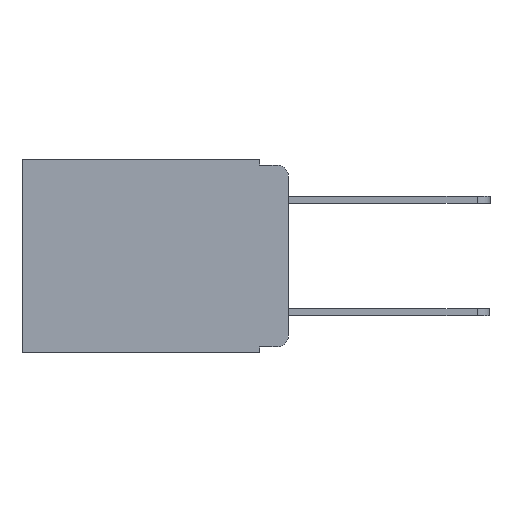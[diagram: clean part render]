
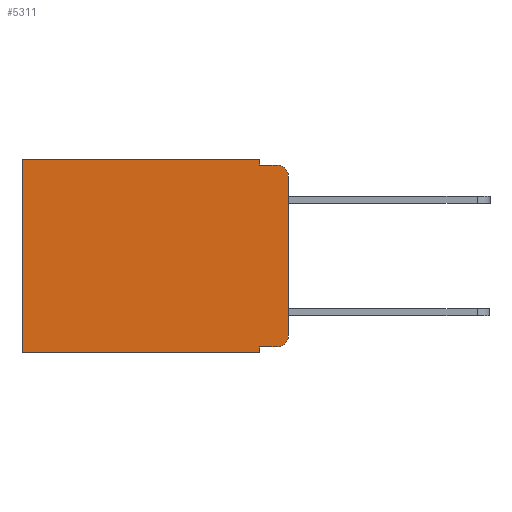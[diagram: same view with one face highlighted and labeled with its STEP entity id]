
A CAD part, left-side view. The second image highlights one B-rep face of the part: STEP entity #5311.
In plain terms, the highlighted planar face has unit normal (-1, 0, 0).
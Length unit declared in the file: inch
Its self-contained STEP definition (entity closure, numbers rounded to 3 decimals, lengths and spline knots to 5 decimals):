
#105 = ORIENTED_EDGE ( 'NONE', *, *, #3213, .T. ) ;
#122 = CARTESIAN_POINT ( 'NONE',  ( 0.298, 0.02, -0.333 ) ) ;
#184 = ORIENTED_EDGE ( 'NONE', *, *, #7238, .F. ) ;
#425 = ORIENTED_EDGE ( 'NONE', *, *, #9780, .T. ) ;
#528 = CARTESIAN_POINT ( 'NONE',  ( 0.298, 0.051, 0. ) ) ;
#529 = DIRECTION ( 'NONE',  ( 0., 0., -1. ) ) ;
#552 = ORIENTED_EDGE ( 'NONE', *, *, #8776, .F. ) ;
#655 = DIRECTION ( 'NONE',  ( 0., 0., -1. ) ) ;
#945 = ORIENTED_EDGE ( 'NONE', *, *, #9925, .T. ) ;
#1077 = ORIENTED_EDGE ( 'NONE', *, *, #9203, .F. ) ;
#1279 = VECTOR ( 'NONE', #6549, 39.37008 ) ;
#1301 = VECTOR ( 'NONE', #7329, 39.37008 ) ;
#1614 = EDGE_CURVE ( 'NONE', #9041, #2381, #5619, .T. ) ;
#1632 = LINE ( 'NONE', #2335, #6495 ) ;
#1778 = VERTEX_POINT ( 'NONE', #10409 ) ;
#2032 = LINE ( 'NONE', #11807, #4285 ) ;
#2217 = VERTEX_POINT ( 'NONE', #7768 ) ;
#2334 = ORIENTED_EDGE ( 'NONE', *, *, #5636, .T. ) ;
#2335 = CARTESIAN_POINT ( 'NONE',  ( 0.298, 0.051, 0. ) ) ;
#2381 = VERTEX_POINT ( 'NONE', #10633 ) ;
#2406 = AXIS2_PLACEMENT_3D ( 'NONE', #9473, #9504, #4091 ) ;
#2476 = VECTOR ( 'NONE', #6270, 39.37008 ) ;
#2969 = ORIENTED_EDGE ( 'NONE', *, *, #1614, .F. ) ;
#2972 = ORIENTED_EDGE ( 'NONE', *, *, #9339, .F. ) ;
#3111 = LINE ( 'NONE', #8207, #10312 ) ;
#3213 = EDGE_CURVE ( 'NONE', #12043, #4428, #3964, .T. ) ;
#3323 = DIRECTION ( 'NONE',  ( 0., 0., -1. ) ) ;
#3486 = CARTESIAN_POINT ( 'NONE',  ( 0.298, 0., 0. ) ) ;
#3513 = CIRCLE ( 'NONE', #10427, 0.02 ) ;
#3964 = LINE ( 'NONE', #3486, #1279 ) ;
#3982 = LINE ( 'NONE', #528, #1301 ) ;
#4091 = DIRECTION ( 'NONE',  ( 0., 0., -1. ) ) ;
#4285 = VECTOR ( 'NONE', #4687, 39.37008 ) ;
#4428 = VERTEX_POINT ( 'NONE', #7315 ) ;
#4435 = DIRECTION ( 'NONE',  ( 0., 1., 0. ) ) ;
#4531 = CARTESIAN_POINT ( 'NONE',  ( 0.298, 0.02, -0.03 ) ) ;
#4687 = DIRECTION ( 'NONE',  ( 0., -1., 0. ) ) ;
#5068 = CARTESIAN_POINT ( 'NONE',  ( 0.298, 0.051, -0.343 ) ) ;
#5310 = LINE ( 'NONE', #9744, #2476 ) ;
#5311 = ADVANCED_FACE ( 'NONE', ( #10951 ), #12104, .F. ) ;
#5364 = AXIS2_PLACEMENT_3D ( 'NONE', #11672, #6459, #529 ) ;
#5519 = DIRECTION ( 'NONE',  ( 0., 0., -1. ) ) ;
#5619 = LINE ( 'NONE', #6500, #10027 ) ;
#5636 = EDGE_CURVE ( 'NONE', #11050, #2381, #10247, .T. ) ;
#6270 = DIRECTION ( 'NONE',  ( 0., 0., -1. ) ) ;
#6459 = DIRECTION ( 'NONE',  ( -1., 0., 0. ) ) ;
#6495 = VECTOR ( 'NONE', #3323, 39.37008 ) ;
#6500 = CARTESIAN_POINT ( 'NONE',  ( 0.298, 0., 0. ) ) ;
#6549 = DIRECTION ( 'NONE',  ( 0., 1., 0. ) ) ;
#7211 = CARTESIAN_POINT ( 'NONE',  ( 0.298, 0., -0.343 ) ) ;
#7238 = EDGE_CURVE ( 'NONE', #9681, #12063, #8993, .T. ) ;
#7286 = CARTESIAN_POINT ( 'NONE',  ( 0.298, 0.051, 0. ) ) ;
#7315 = CARTESIAN_POINT ( 'NONE',  ( 0.298, 0.473, 0. ) ) ;
#7329 = DIRECTION ( 'NONE',  ( 0., 0., -1. ) ) ;
#7437 = EDGE_CURVE ( 'NONE', #2217, #11050, #2032, .T. ) ;
#7768 = CARTESIAN_POINT ( 'NONE',  ( 0.298, 0.051, -0.333 ) ) ;
#8171 = CARTESIAN_POINT ( 'NONE',  ( 0.298, 0.473, -0.343 ) ) ;
#8207 = CARTESIAN_POINT ( 'NONE',  ( 0.298, 0.051, -0.01 ) ) ;
#8595 = ORIENTED_EDGE ( 'NONE', *, *, #7437, .T. ) ;
#8776 = EDGE_CURVE ( 'NONE', #12043, #9581, #3982, .T. ) ;
#8993 = LINE ( 'NONE', #7211, #11037 ) ;
#9041 = VERTEX_POINT ( 'NONE', #9429 ) ;
#9203 = EDGE_CURVE ( 'NONE', #2217, #9681, #1632, .T. ) ;
#9339 = EDGE_CURVE ( 'NONE', #9581, #1778, #3111, .T. ) ;
#9429 = CARTESIAN_POINT ( 'NONE',  ( 0.298, 0., -0.03 ) ) ;
#9473 = CARTESIAN_POINT ( 'NONE',  ( 0.298, 0., 0. ) ) ;
#9504 = DIRECTION ( 'NONE',  ( 1., 0., 0. ) ) ;
#9581 = VERTEX_POINT ( 'NONE', #11181 ) ;
#9681 = VERTEX_POINT ( 'NONE', #5068 ) ;
#9744 = CARTESIAN_POINT ( 'NONE',  ( 0.298, 0.473, 0. ) ) ;
#9780 = EDGE_CURVE ( 'NONE', #4428, #12063, #5310, .T. ) ;
#9925 = EDGE_CURVE ( 'NONE', #9041, #1778, #3513, .T. ) ;
#9953 = DIRECTION ( 'NONE',  ( 0., -1., 0. ) ) ;
#10027 = VECTOR ( 'NONE', #655, 39.37008 ) ;
#10247 = CIRCLE ( 'NONE', #5364, 0.02 ) ;
#10273 = EDGE_LOOP ( 'NONE', ( #2969, #945, #2972, #552, #105, #425, #184, #1077, #8595, #2334 ) ) ;
#10312 = VECTOR ( 'NONE', #9953, 39.37008 ) ;
#10409 = CARTESIAN_POINT ( 'NONE',  ( 0.298, 0.02, -0.01 ) ) ;
#10427 = AXIS2_PLACEMENT_3D ( 'NONE', #4531, #10806, #5519 ) ;
#10633 = CARTESIAN_POINT ( 'NONE',  ( 0.298, 0., -0.313 ) ) ;
#10806 = DIRECTION ( 'NONE',  ( -1., 0., 0. ) ) ;
#10951 = FACE_OUTER_BOUND ( 'NONE', #10273, .T. ) ;
#11037 = VECTOR ( 'NONE', #4435, 39.37008 ) ;
#11050 = VERTEX_POINT ( 'NONE', #122 ) ;
#11181 = CARTESIAN_POINT ( 'NONE',  ( 0.298, 0.051, -0.01 ) ) ;
#11672 = CARTESIAN_POINT ( 'NONE',  ( 0.298, 0.02, -0.313 ) ) ;
#11807 = CARTESIAN_POINT ( 'NONE',  ( 0.298, 0.051, -0.333 ) ) ;
#12043 = VERTEX_POINT ( 'NONE', #7286 ) ;
#12063 = VERTEX_POINT ( 'NONE', #8171 ) ;
#12104 = PLANE ( 'NONE',  #2406 ) ;
